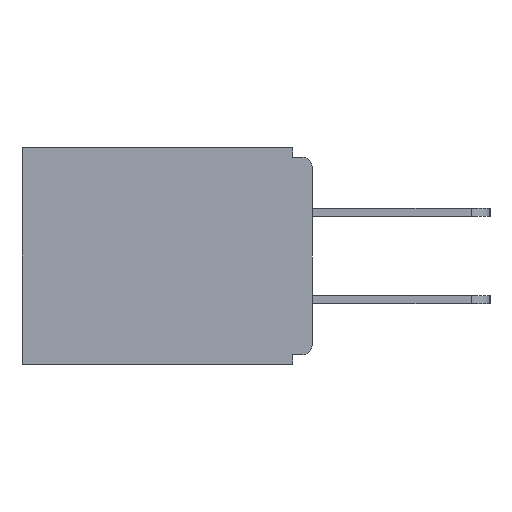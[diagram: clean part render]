
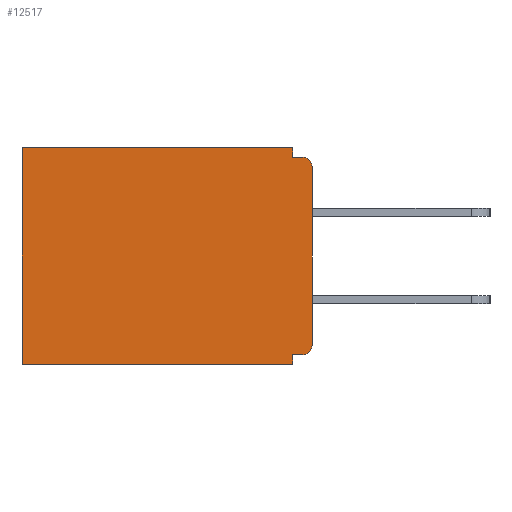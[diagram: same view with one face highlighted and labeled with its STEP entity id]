
A CAD part, left-side view. The second image highlights one B-rep face of the part: STEP entity #12517.
In plain terms, the highlighted planar face has unit normal (-1, 0, 0).
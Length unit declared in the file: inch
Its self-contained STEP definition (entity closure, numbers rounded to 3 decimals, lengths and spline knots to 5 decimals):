
#118 = VERTEX_POINT ( 'NONE', #18596 ) ;
#238 = EDGE_CURVE ( 'NONE', #11515, #8556, #8067, .T. ) ;
#244 = VECTOR ( 'NONE', #12114, 39.37008 ) ;
#256 = LINE ( 'NONE', #3852, #4159 ) ;
#313 = LINE ( 'NONE', #16437, #13385 ) ;
#713 = AXIS2_PLACEMENT_3D ( 'NONE', #5376, #17834, #14160 ) ;
#1449 = ORIENTED_EDGE ( 'NONE', *, *, #14777, .F. ) ;
#1658 = EDGE_CURVE ( 'NONE', #11515, #118, #7194, .T. ) ;
#1733 = ORIENTED_EDGE ( 'NONE', *, *, #20937, .F. ) ;
#2090 = VERTEX_POINT ( 'NONE', #16707 ) ;
#2186 = CIRCLE ( 'NONE', #17481, 0.015 ) ;
#2215 = VECTOR ( 'NONE', #22542, 39.37008 ) ;
#2343 = DIRECTION ( 'NONE',  ( 0., 1., 0. ) ) ;
#2644 = CARTESIAN_POINT ( 'NONE',  ( 0.298, 0., -0.015 ) ) ;
#2709 = CARTESIAN_POINT ( 'NONE',  ( 0.298, 0., -0.343 ) ) ;
#2905 = CARTESIAN_POINT ( 'NONE',  ( 0.298, 0.015, -0.03 ) ) ;
#3065 = CARTESIAN_POINT ( 'NONE',  ( 0.298, 0., -0.313 ) ) ;
#3836 = CARTESIAN_POINT ( 'NONE',  ( 0.298, 0.031, -0.328 ) ) ;
#3852 = CARTESIAN_POINT ( 'NONE',  ( 0.298, 0.46, 0. ) ) ;
#4159 = VECTOR ( 'NONE', #14569, 39.37008 ) ;
#4167 = VECTOR ( 'NONE', #2343, 39.37008 ) ;
#4432 = VECTOR ( 'NONE', #13467, 39.37008 ) ;
#4493 = VECTOR ( 'NONE', #17111, 39.37008 ) ;
#4713 = DIRECTION ( 'NONE',  ( -1., 0., 0. ) ) ;
#4785 = DIRECTION ( 'NONE',  ( 0., 0., -1. ) ) ;
#5082 = CARTESIAN_POINT ( 'NONE',  ( 0.298, 0., -0.03 ) ) ;
#5376 = CARTESIAN_POINT ( 'NONE',  ( 0.298, 0.015, -0.313 ) ) ;
#5915 = VERTEX_POINT ( 'NONE', #5082 ) ;
#6778 = ORIENTED_EDGE ( 'NONE', *, *, #19272, .T. ) ;
#7194 = LINE ( 'NONE', #9315, #20863 ) ;
#8067 = LINE ( 'NONE', #17231, #4432 ) ;
#8556 = VERTEX_POINT ( 'NONE', #22985 ) ;
#8844 = CIRCLE ( 'NONE', #713, 0.015 ) ;
#9230 = AXIS2_PLACEMENT_3D ( 'NONE', #22578, #20679, #9922 ) ;
#9315 = CARTESIAN_POINT ( 'NONE',  ( 0.298, 0.031, -0.343 ) ) ;
#9415 = CARTESIAN_POINT ( 'NONE',  ( 0.298, 0.015, -0.328 ) ) ;
#9922 = DIRECTION ( 'NONE',  ( 0., 0., -1. ) ) ;
#11515 = VERTEX_POINT ( 'NONE', #14220 ) ;
#11953 = ORIENTED_EDGE ( 'NONE', *, *, #20239, .T. ) ;
#12114 = DIRECTION ( 'NONE',  ( 0., 1., 0. ) ) ;
#12487 = LINE ( 'NONE', #2709, #244 ) ;
#12517 = ADVANCED_FACE ( 'NONE', ( #14135 ), #17070, .F. ) ;
#12936 = VERTEX_POINT ( 'NONE', #3836 ) ;
#13256 = ORIENTED_EDGE ( 'NONE', *, *, #17655, .F. ) ;
#13385 = VECTOR ( 'NONE', #21689, 39.37008 ) ;
#13467 = DIRECTION ( 'NONE',  ( 0., 1., 0. ) ) ;
#13636 = EDGE_CURVE ( 'NONE', #13928, #12936, #20625, .T. ) ;
#13928 = VERTEX_POINT ( 'NONE', #9415 ) ;
#14135 = FACE_OUTER_BOUND ( 'NONE', #16568, .T. ) ;
#14160 = DIRECTION ( 'NONE',  ( 0., 0., -1. ) ) ;
#14219 = VERTEX_POINT ( 'NONE', #19243 ) ;
#14220 = CARTESIAN_POINT ( 'NONE',  ( 0.298, 0.031, 0. ) ) ;
#14262 = ORIENTED_EDGE ( 'NONE', *, *, #238, .T. ) ;
#14530 = CARTESIAN_POINT ( 'NONE',  ( 0.298, 0., -0.328 ) ) ;
#14569 = DIRECTION ( 'NONE',  ( 0., 0., -1. ) ) ;
#14777 = EDGE_CURVE ( 'NONE', #21273, #14219, #12487, .T. ) ;
#14864 = DIRECTION ( 'NONE',  ( 0., 0., -1. ) ) ;
#14929 = VERTEX_POINT ( 'NONE', #3065 ) ;
#14966 = EDGE_CURVE ( 'NONE', #5915, #2090, #2186, .T. ) ;
#15060 = CARTESIAN_POINT ( 'NONE',  ( 0.298, 0.031, -0.343 ) ) ;
#15210 = ORIENTED_EDGE ( 'NONE', *, *, #20010, .F. ) ;
#16437 = CARTESIAN_POINT ( 'NONE',  ( 0.298, 0., 0. ) ) ;
#16568 = EDGE_LOOP ( 'NONE', ( #21121, #1733, #20198, #14262, #6778, #1449, #15210, #17896, #11953, #13256 ) ) ;
#16707 = CARTESIAN_POINT ( 'NONE',  ( 0.298, 0.015, -0.015 ) ) ;
#17070 = PLANE ( 'NONE',  #9230 ) ;
#17111 = DIRECTION ( 'NONE',  ( 0., 0., -1. ) ) ;
#17231 = CARTESIAN_POINT ( 'NONE',  ( 0.298, 0., 0. ) ) ;
#17333 = LINE ( 'NONE', #15060, #4493 ) ;
#17481 = AXIS2_PLACEMENT_3D ( 'NONE', #2905, #4713, #4785 ) ;
#17655 = EDGE_CURVE ( 'NONE', #5915, #14929, #313, .T. ) ;
#17834 = DIRECTION ( 'NONE',  ( -1., 0., 0. ) ) ;
#17896 = ORIENTED_EDGE ( 'NONE', *, *, #13636, .F. ) ;
#18596 = CARTESIAN_POINT ( 'NONE',  ( 0.298, 0.031, -0.015 ) ) ;
#19243 = CARTESIAN_POINT ( 'NONE',  ( 0.298, 0.46, -0.343 ) ) ;
#19272 = EDGE_CURVE ( 'NONE', #8556, #14219, #256, .T. ) ;
#19559 = CARTESIAN_POINT ( 'NONE',  ( 0.298, 0.031, -0.343 ) ) ;
#20010 = EDGE_CURVE ( 'NONE', #12936, #21273, #17333, .T. ) ;
#20198 = ORIENTED_EDGE ( 'NONE', *, *, #1658, .F. ) ;
#20239 = EDGE_CURVE ( 'NONE', #13928, #14929, #8844, .T. ) ;
#20625 = LINE ( 'NONE', #14530, #4167 ) ;
#20679 = DIRECTION ( 'NONE',  ( 1., 0., 0. ) ) ;
#20863 = VECTOR ( 'NONE', #14864, 39.37008 ) ;
#20937 = EDGE_CURVE ( 'NONE', #118, #2090, #21724, .T. ) ;
#21121 = ORIENTED_EDGE ( 'NONE', *, *, #14966, .T. ) ;
#21273 = VERTEX_POINT ( 'NONE', #19559 ) ;
#21689 = DIRECTION ( 'NONE',  ( 0., 0., -1. ) ) ;
#21724 = LINE ( 'NONE', #2644, #2215 ) ;
#22542 = DIRECTION ( 'NONE',  ( 0., -1., 0. ) ) ;
#22578 = CARTESIAN_POINT ( 'NONE',  ( 0.298, 0., 0. ) ) ;
#22985 = CARTESIAN_POINT ( 'NONE',  ( 0.298, 0.46, 0. ) ) ;
